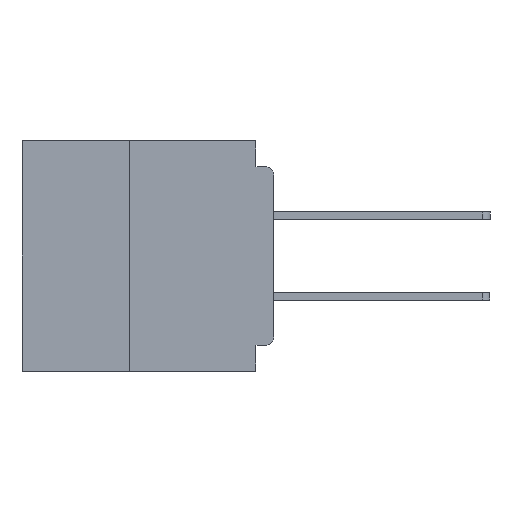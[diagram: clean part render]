
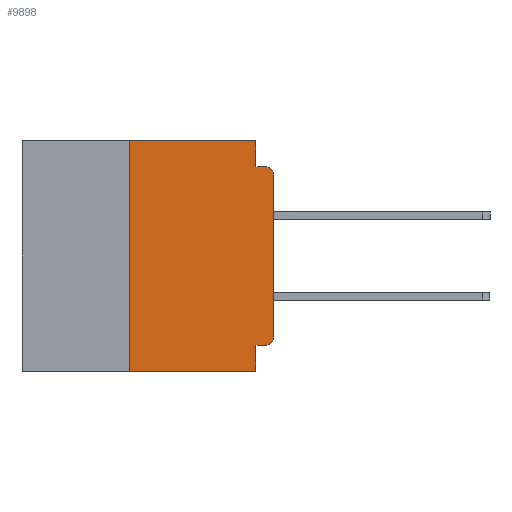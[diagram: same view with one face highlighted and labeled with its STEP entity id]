
A CAD part, left-side view. The second image highlights one B-rep face of the part: STEP entity #9898.
In plain terms, the highlighted planar face has unit normal (-1, 0, 0).
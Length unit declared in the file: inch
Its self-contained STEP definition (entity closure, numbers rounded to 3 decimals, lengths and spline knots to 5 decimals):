
#208 = EDGE_CURVE ( 'NONE', #34152, #16868, #43211, .T. ) ;
#524 = EDGE_CURVE ( 'NONE', #9886, #40905, #40606, .T. ) ;
#814 = VECTOR ( 'NONE', #35886, 39.37008 ) ;
#1017 = EDGE_CURVE ( 'NONE', #5348, #23900, #39517, .T. ) ;
#1157 = VECTOR ( 'NONE', #15367, 39.37008 ) ;
#1284 = ORIENTED_EDGE ( 'NONE', *, *, #524, .F. ) ;
#1947 = VERTEX_POINT ( 'NONE', #36870 ) ;
#3307 = LINE ( 'NONE', #31907, #1157 ) ;
#3498 = CARTESIAN_POINT ( 'NONE',  ( 0., 0.015, -0.06 ) ) ;
#3514 = CARTESIAN_POINT ( 'NONE',  ( 0., 0.437, 0. ) ) ;
#3673 = PLANE ( 'NONE',  #11599 ) ;
#3945 = EDGE_LOOP ( 'NONE', ( #34546, #13815, #1284, #15405, #25440, #40569, #30810, #31080, #40520, #36516 ) ) ;
#5348 = VERTEX_POINT ( 'NONE', #19877 ) ;
#5645 = CARTESIAN_POINT ( 'NONE',  ( 0., 0.031, 0. ) ) ;
#6997 = DIRECTION ( 'NONE',  ( 0., 0., -1. ) ) ;
#7177 = DIRECTION ( 'NONE',  ( 1., 0., 0. ) ) ;
#7211 = EDGE_CURVE ( 'NONE', #5348, #1947, #33017, .T. ) ;
#8156 = VECTOR ( 'NONE', #19921, 39.37008 ) ;
#8404 = CARTESIAN_POINT ( 'NONE',  ( 0., 0., -0.06 ) ) ;
#9886 = VERTEX_POINT ( 'NONE', #40363 ) ;
#9898 = ADVANCED_FACE ( 'NONE', ( #28725 ), #3673, .F. ) ;
#11599 = AXIS2_PLACEMENT_3D ( 'NONE', #3514, #7177, #30437 ) ;
#13359 = CARTESIAN_POINT ( 'NONE',  ( 0., 0., -0.34 ) ) ;
#13815 = ORIENTED_EDGE ( 'NONE', *, *, #30283, .T. ) ;
#14326 = VECTOR ( 'NONE', #24111, 39.37008 ) ;
#15367 = DIRECTION ( 'NONE',  ( 0., -1., 0. ) ) ;
#15405 = ORIENTED_EDGE ( 'NONE', *, *, #28179, .F. ) ;
#15638 = DIRECTION ( 'NONE',  ( 0., -1., 0. ) ) ;
#15681 = CARTESIAN_POINT ( 'NONE',  ( 0., 0., -0.045 ) ) ;
#15712 = CARTESIAN_POINT ( 'NONE',  ( 0., 0.25, -0.4 ) ) ;
#16602 = CARTESIAN_POINT ( 'NONE',  ( 0., 0.25, -0.4 ) ) ;
#16668 = EDGE_CURVE ( 'NONE', #27633, #34152, #33653, .T. ) ;
#16868 = VERTEX_POINT ( 'NONE', #24243 ) ;
#16891 = EDGE_CURVE ( 'NONE', #1947, #40718, #42984, .T. ) ;
#18488 = VECTOR ( 'NONE', #19127, 39.37008 ) ;
#18600 = CARTESIAN_POINT ( 'NONE',  ( 0., 0.031, -0.4 ) ) ;
#19127 = DIRECTION ( 'NONE',  ( 0., 0., -1. ) ) ;
#19877 = CARTESIAN_POINT ( 'NONE',  ( 0., 0.015, -0.355 ) ) ;
#19921 = DIRECTION ( 'NONE',  ( 0., 0., 1. ) ) ;
#21049 = CARTESIAN_POINT ( 'NONE',  ( 0., 0.031, -0.4 ) ) ;
#22124 = CARTESIAN_POINT ( 'NONE',  ( 0., 0.015, -0.34 ) ) ;
#22348 = DIRECTION ( 'NONE',  ( -1., 0., 0. ) ) ;
#22435 = CIRCLE ( 'NONE', #39083, 0.015 ) ;
#22775 = EDGE_CURVE ( 'NONE', #23900, #31931, #33033, .T. ) ;
#23900 = VERTEX_POINT ( 'NONE', #13359 ) ;
#24111 = DIRECTION ( 'NONE',  ( 0., 1., 0. ) ) ;
#24243 = CARTESIAN_POINT ( 'NONE',  ( 0., 0.031, 0. ) ) ;
#25190 = VECTOR ( 'NONE', #39202, 39.37008 ) ;
#25440 = ORIENTED_EDGE ( 'NONE', *, *, #208, .F. ) ;
#25935 = CARTESIAN_POINT ( 'NONE',  ( 0., 0., 0. ) ) ;
#26930 = DIRECTION ( 'NONE',  ( -1., 0., 0. ) ) ;
#27312 = LINE ( 'NONE', #5645, #18488 ) ;
#27574 = DIRECTION ( 'NONE',  ( 0., 0., -1. ) ) ;
#27633 = VERTEX_POINT ( 'NONE', #15712 ) ;
#28179 = EDGE_CURVE ( 'NONE', #16868, #9886, #27312, .T. ) ;
#28725 = FACE_OUTER_BOUND ( 'NONE', #3945, .T. ) ;
#30283 = EDGE_CURVE ( 'NONE', #31931, #40905, #22435, .T. ) ;
#30437 = DIRECTION ( 'NONE',  ( 0., 0., -1. ) ) ;
#30810 = ORIENTED_EDGE ( 'NONE', *, *, #32623, .T. ) ;
#31080 = ORIENTED_EDGE ( 'NONE', *, *, #16891, .F. ) ;
#31907 = CARTESIAN_POINT ( 'NONE',  ( 0., 0.437, -0.4 ) ) ;
#31931 = VERTEX_POINT ( 'NONE', #8404 ) ;
#32623 = EDGE_CURVE ( 'NONE', #27633, #40718, #3307, .T. ) ;
#32812 = VECTOR ( 'NONE', #15638, 39.37008 ) ;
#32842 = CARTESIAN_POINT ( 'NONE',  ( 0., 0.015, -0.045 ) ) ;
#33017 = LINE ( 'NONE', #34175, #14326 ) ;
#33033 = LINE ( 'NONE', #25935, #25190 ) ;
#33059 = AXIS2_PLACEMENT_3D ( 'NONE', #22124, #22348, #39626 ) ;
#33653 = LINE ( 'NONE', #16602, #8156 ) ;
#34152 = VERTEX_POINT ( 'NONE', #43393 ) ;
#34174 = VECTOR ( 'NONE', #27574, 39.37008 ) ;
#34175 = CARTESIAN_POINT ( 'NONE',  ( 0., 0., -0.355 ) ) ;
#34546 = ORIENTED_EDGE ( 'NONE', *, *, #22775, .T. ) ;
#35886 = DIRECTION ( 'NONE',  ( 0., -1., 0. ) ) ;
#36381 = CARTESIAN_POINT ( 'NONE',  ( 0., 0.437, 0. ) ) ;
#36516 = ORIENTED_EDGE ( 'NONE', *, *, #1017, .T. ) ;
#36870 = CARTESIAN_POINT ( 'NONE',  ( 0., 0.031, -0.355 ) ) ;
#39083 = AXIS2_PLACEMENT_3D ( 'NONE', #3498, #26930, #6997 ) ;
#39202 = DIRECTION ( 'NONE',  ( 0., 0., 1. ) ) ;
#39517 = CIRCLE ( 'NONE', #33059, 0.015 ) ;
#39626 = DIRECTION ( 'NONE',  ( 0., 0., -1. ) ) ;
#40363 = CARTESIAN_POINT ( 'NONE',  ( 0., 0.031, -0.045 ) ) ;
#40520 = ORIENTED_EDGE ( 'NONE', *, *, #7211, .F. ) ;
#40569 = ORIENTED_EDGE ( 'NONE', *, *, #16668, .F. ) ;
#40606 = LINE ( 'NONE', #15681, #32812 ) ;
#40718 = VERTEX_POINT ( 'NONE', #18600 ) ;
#40905 = VERTEX_POINT ( 'NONE', #32842 ) ;
#42984 = LINE ( 'NONE', #21049, #34174 ) ;
#43211 = LINE ( 'NONE', #36381, #814 ) ;
#43393 = CARTESIAN_POINT ( 'NONE',  ( 0., 0.25, 0. ) ) ;
